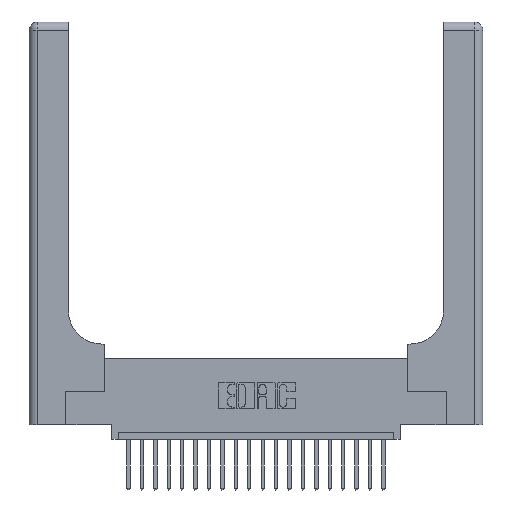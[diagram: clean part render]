
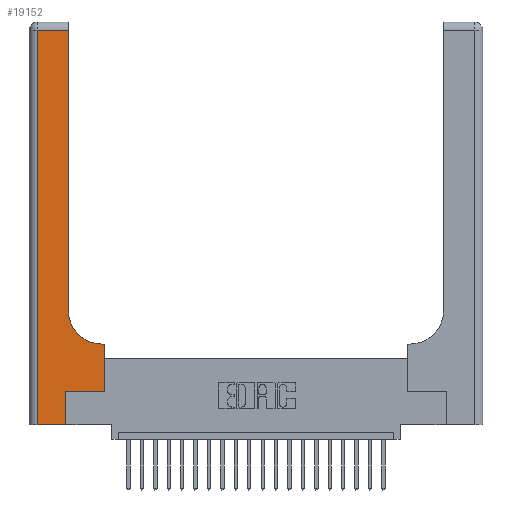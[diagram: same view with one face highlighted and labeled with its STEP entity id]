
A CAD part, top view. The second image highlights one B-rep face of the part: STEP entity #19152.
In plain terms, the highlighted planar face has unit normal (0, 0, 1).
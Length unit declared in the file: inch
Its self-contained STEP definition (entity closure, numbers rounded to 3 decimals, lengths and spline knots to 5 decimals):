
#420 = CARTESIAN_POINT ( 'NONE',  ( 0.269, 0.25, 0.37 ) ) ;
#537 = ORIENTED_EDGE ( 'NONE', *, *, #1415, .T. ) ;
#616 = EDGE_CURVE ( 'NONE', #2782, #12749, #2509, .T. ) ;
#773 = LINE ( 'NONE', #22643, #1615 ) ;
#976 = VECTOR ( 'NONE', #14141, 39.37008 ) ;
#1415 = EDGE_CURVE ( 'NONE', #9026, #18294, #773, .T. ) ;
#1428 = VERTEX_POINT ( 'NONE', #11853 ) ;
#1546 = LINE ( 'NONE', #23124, #976 ) ;
#1577 = PLANE ( 'NONE',  #9332 ) ;
#1615 = VECTOR ( 'NONE', #6530, 39.37008 ) ;
#1838 = LINE ( 'NONE', #12629, #6103 ) ;
#2110 = ORIENTED_EDGE ( 'NONE', *, *, #7723, .T. ) ;
#2509 = LINE ( 'NONE', #2722, #11273 ) ;
#2673 = CARTESIAN_POINT ( 'NONE',  ( 0.269, 0., 0.37 ) ) ;
#2722 = CARTESIAN_POINT ( 'NONE',  ( 0.06, 3., 0.37 ) ) ;
#2782 = VERTEX_POINT ( 'NONE', #20428 ) ;
#3310 = EDGE_CURVE ( 'NONE', #17503, #19739, #5222, .T. ) ;
#3816 = DIRECTION ( 'NONE',  ( 1., 0., 0. ) ) ;
#3911 = VECTOR ( 'NONE', #3816, 39.37008 ) ;
#4128 = EDGE_CURVE ( 'NONE', #19739, #1428, #22270, .T. ) ;
#5222 = LINE ( 'NONE', #17663, #17587 ) ;
#5441 = ORIENTED_EDGE ( 'NONE', *, *, #19634, .T. ) ;
#6103 = VECTOR ( 'NONE', #18204, 39.37008 ) ;
#6530 = DIRECTION ( 'NONE',  ( 1., 0., 0. ) ) ;
#7444 = CARTESIAN_POINT ( 'NONE',  ( 0., 3., 0.37 ) ) ;
#7462 = DIRECTION ( 'NONE',  ( 0., 1., 0. ) ) ;
#7522 = DIRECTION ( 'NONE',  ( -1., 0., 0. ) ) ;
#7723 = EDGE_CURVE ( 'NONE', #19582, #2782, #1546, .T. ) ;
#9026 = VERTEX_POINT ( 'NONE', #420 ) ;
#9332 = AXIS2_PLACEMENT_3D ( 'NONE', #7444, #21788, #7522 ) ;
#9425 = ORIENTED_EDGE ( 'NONE', *, *, #17611, .T. ) ;
#9795 = VERTEX_POINT ( 'NONE', #2673 ) ;
#10475 = CARTESIAN_POINT ( 'NONE',  ( 0.5585, 0.25, 0.37 ) ) ;
#11273 = VECTOR ( 'NONE', #19018, 39.37008 ) ;
#11542 = LINE ( 'NONE', #19729, #12933 ) ;
#11839 = AXIS2_PLACEMENT_3D ( 'NONE', #15221, #18831, #13388 ) ;
#11853 = CARTESIAN_POINT ( 'NONE',  ( 0.2915, 0.85, 0.37 ) ) ;
#12496 = CARTESIAN_POINT ( 'NONE',  ( 0., 0., 0.37 ) ) ;
#12629 = CARTESIAN_POINT ( 'NONE',  ( 0.5585, 0.25, 0.37 ) ) ;
#12749 = VERTEX_POINT ( 'NONE', #22363 ) ;
#12769 = LINE ( 'NONE', #15623, #15033 ) ;
#12933 = VECTOR ( 'NONE', #7462, 39.37008 ) ;
#13031 = FACE_OUTER_BOUND ( 'NONE', #20713, .T. ) ;
#13388 = DIRECTION ( 'NONE',  ( 1., 0., 0. ) ) ;
#14002 = ORIENTED_EDGE ( 'NONE', *, *, #4128, .T. ) ;
#14141 = DIRECTION ( 'NONE',  ( -1., 0., 0. ) ) ;
#14162 = EDGE_CURVE ( 'NONE', #12749, #9795, #15225, .T. ) ;
#14202 = EDGE_CURVE ( 'NONE', #9795, #9026, #11542, .T. ) ;
#14559 = ORIENTED_EDGE ( 'NONE', *, *, #616, .T. ) ;
#15033 = VECTOR ( 'NONE', #19479, 39.37008 ) ;
#15221 = CARTESIAN_POINT ( 'NONE',  ( 0.5415, 0.85, 0.37 ) ) ;
#15225 = LINE ( 'NONE', #12496, #3911 ) ;
#15603 = CARTESIAN_POINT ( 'NONE',  ( 0.5585, 0.6, 0.37 ) ) ;
#15623 = CARTESIAN_POINT ( 'NONE',  ( 0.2915, 3., 0.37 ) ) ;
#17067 = ORIENTED_EDGE ( 'NONE', *, *, #14202, .T. ) ;
#17503 = VERTEX_POINT ( 'NONE', #15603 ) ;
#17587 = VECTOR ( 'NONE', #22014, 39.37008 ) ;
#17611 = EDGE_CURVE ( 'NONE', #18294, #17503, #1838, .T. ) ;
#17663 = CARTESIAN_POINT ( 'NONE',  ( 0.2915, 0.6, 0.37 ) ) ;
#18204 = DIRECTION ( 'NONE',  ( 0., 1., 0. ) ) ;
#18294 = VERTEX_POINT ( 'NONE', #10475 ) ;
#18831 = DIRECTION ( 'NONE',  ( 0., 0., -1. ) ) ;
#19018 = DIRECTION ( 'NONE',  ( 0., -1., 0. ) ) ;
#19152 = ADVANCED_FACE ( 'NONE', ( #13031 ), #1577, .F. ) ;
#19161 = CARTESIAN_POINT ( 'NONE',  ( 0.5415, 0.6, 0.37 ) ) ;
#19288 = ORIENTED_EDGE ( 'NONE', *, *, #14162, .T. ) ;
#19479 = DIRECTION ( 'NONE',  ( 0., 1., 0. ) ) ;
#19582 = VERTEX_POINT ( 'NONE', #23305 ) ;
#19634 = EDGE_CURVE ( 'NONE', #1428, #19582, #12769, .T. ) ;
#19729 = CARTESIAN_POINT ( 'NONE',  ( 0.269, 0., 0.37 ) ) ;
#19739 = VERTEX_POINT ( 'NONE', #19161 ) ;
#20428 = CARTESIAN_POINT ( 'NONE',  ( 0.06, 2.94, 0.37 ) ) ;
#20713 = EDGE_LOOP ( 'NONE', ( #5441, #2110, #14559, #19288, #17067, #537, #9425, #20800, #14002 ) ) ;
#20800 = ORIENTED_EDGE ( 'NONE', *, *, #3310, .T. ) ;
#21788 = DIRECTION ( 'NONE',  ( 0., 0., -1. ) ) ;
#22014 = DIRECTION ( 'NONE',  ( -1., 0., 0. ) ) ;
#22270 = CIRCLE ( 'NONE', #11839, 0.25 ) ;
#22363 = CARTESIAN_POINT ( 'NONE',  ( 0.06, 0., 0.37 ) ) ;
#22643 = CARTESIAN_POINT ( 'NONE',  ( 0.269, 0.25, 0.37 ) ) ;
#23124 = CARTESIAN_POINT ( 'NONE',  ( 0., 2.94, 0.37 ) ) ;
#23305 = CARTESIAN_POINT ( 'NONE',  ( 0.2915, 2.94, 0.37 ) ) ;
